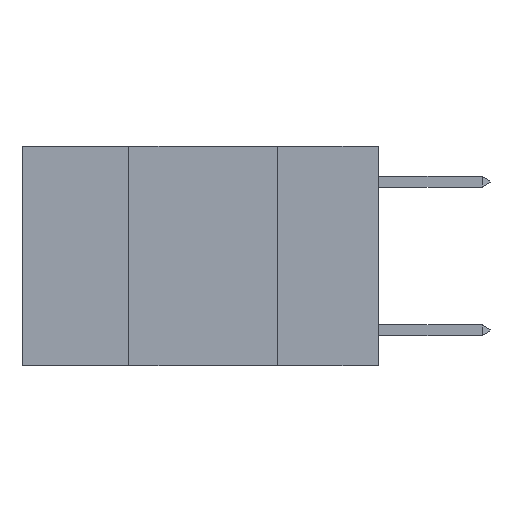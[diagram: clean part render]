
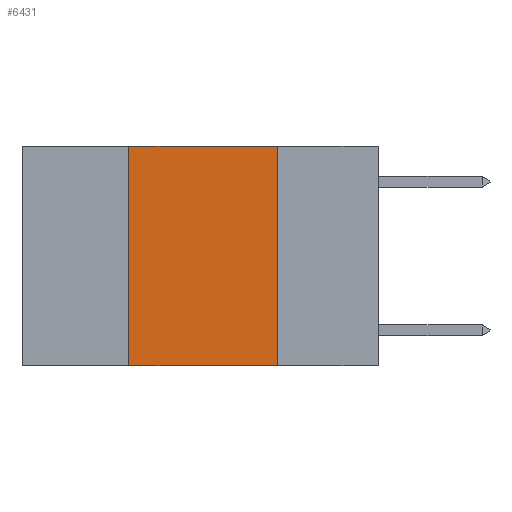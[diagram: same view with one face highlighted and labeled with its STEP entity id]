
A CAD part, left-side view. The second image highlights one B-rep face of the part: STEP entity #6431.
In plain terms, the highlighted planar face has unit normal (-1, 0, 0).
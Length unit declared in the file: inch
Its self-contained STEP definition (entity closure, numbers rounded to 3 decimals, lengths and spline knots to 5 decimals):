
#180 = CARTESIAN_POINT ( 'NONE',  ( 0., 0.42, 0. ) ) ;
#257 = EDGE_CURVE ( 'NONE', #5264, #14231, #9787, .T. ) ;
#421 = EDGE_CURVE ( 'NONE', #7516, #6346, #6535, .T. ) ;
#569 = CARTESIAN_POINT ( 'NONE',  ( 0., 0.42, -0.37 ) ) ;
#1363 = ORIENTED_EDGE ( 'NONE', *, *, #257, .F. ) ;
#2474 = CARTESIAN_POINT ( 'NONE',  ( 0., 0.6, 0. ) ) ;
#2606 = CARTESIAN_POINT ( 'NONE',  ( 0., 0.6, -0.37 ) ) ;
#2697 = VECTOR ( 'NONE', #11780, 39.37008 ) ;
#2862 = DIRECTION ( 'NONE',  ( 0., 0., -1. ) ) ;
#3149 = EDGE_LOOP ( 'NONE', ( #8933, #13459, #1363, #9761 ) ) ;
#3511 = LINE ( 'NONE', #10693, #2697 ) ;
#5264 = VERTEX_POINT ( 'NONE', #569 ) ;
#6071 = DIRECTION ( 'NONE',  ( 0., 0., -1. ) ) ;
#6257 = AXIS2_PLACEMENT_3D ( 'NONE', #2474, #13068, #6071 ) ;
#6346 = VERTEX_POINT ( 'NONE', #7078 ) ;
#6431 = ADVANCED_FACE ( 'NONE', ( #14449 ), #8458, .F. ) ;
#6535 = LINE ( 'NONE', #7856, #8431 ) ;
#6816 = EDGE_CURVE ( 'NONE', #5264, #6346, #9683, .T. ) ;
#7078 = CARTESIAN_POINT ( 'NONE',  ( 0., 0.17, -0.37 ) ) ;
#7516 = VERTEX_POINT ( 'NONE', #8183 ) ;
#7856 = CARTESIAN_POINT ( 'NONE',  ( 0., 0.17, 0. ) ) ;
#7982 = VECTOR ( 'NONE', #8367, 39.37008 ) ;
#8183 = CARTESIAN_POINT ( 'NONE',  ( 0., 0.17, 0. ) ) ;
#8367 = DIRECTION ( 'NONE',  ( 0., -1., 0. ) ) ;
#8431 = VECTOR ( 'NONE', #2862, 39.37008 ) ;
#8458 = PLANE ( 'NONE',  #6257 ) ;
#8933 = ORIENTED_EDGE ( 'NONE', *, *, #421, .F. ) ;
#9683 = LINE ( 'NONE', #2606, #7982 ) ;
#9761 = ORIENTED_EDGE ( 'NONE', *, *, #6816, .T. ) ;
#9787 = LINE ( 'NONE', #180, #13147 ) ;
#10693 = CARTESIAN_POINT ( 'NONE',  ( 0., 0.6, 0. ) ) ;
#10989 = DIRECTION ( 'NONE',  ( 0., 0., 1. ) ) ;
#11780 = DIRECTION ( 'NONE',  ( 0., -1., 0. ) ) ;
#13068 = DIRECTION ( 'NONE',  ( 1., 0., 0. ) ) ;
#13147 = VECTOR ( 'NONE', #10989, 39.37008 ) ;
#13282 = EDGE_CURVE ( 'NONE', #14231, #7516, #3511, .T. ) ;
#13459 = ORIENTED_EDGE ( 'NONE', *, *, #13282, .F. ) ;
#14231 = VERTEX_POINT ( 'NONE', #14332 ) ;
#14332 = CARTESIAN_POINT ( 'NONE',  ( 0., 0.42, 0. ) ) ;
#14449 = FACE_OUTER_BOUND ( 'NONE', #3149, .T. ) ;
